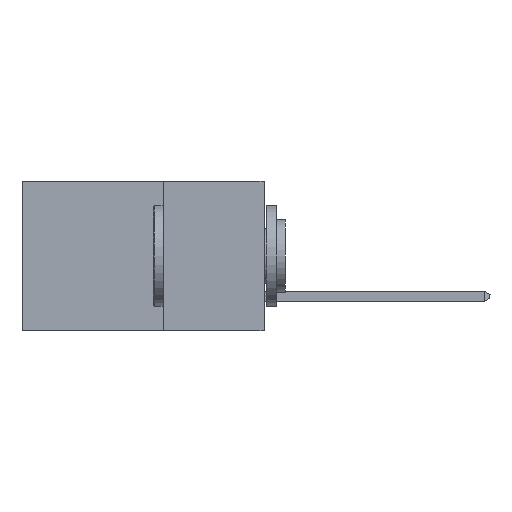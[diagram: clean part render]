
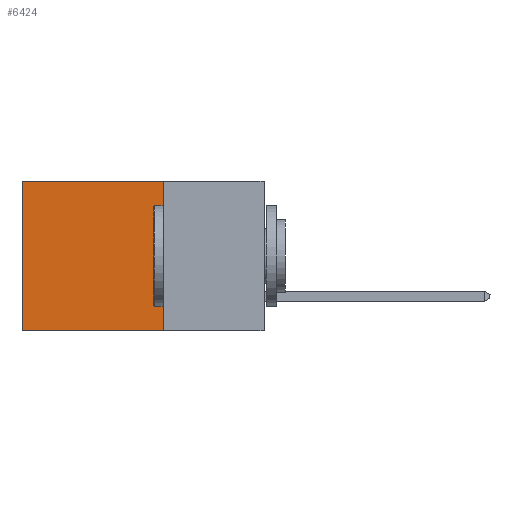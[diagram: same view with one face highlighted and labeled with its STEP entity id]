
A CAD part, left-side view. The second image highlights one B-rep face of the part: STEP entity #6424.
In plain terms, the highlighted planar face has unit normal (-1, 0, 0).
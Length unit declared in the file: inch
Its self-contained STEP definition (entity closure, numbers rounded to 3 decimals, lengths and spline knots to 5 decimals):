
#347 = DIRECTION ( 'NONE',  ( 0., 0., -1. ) ) ;
#1342 = CARTESIAN_POINT ( 'NONE',  ( 0.298, 0.25, -0.37 ) ) ;
#1384 = ORIENTED_EDGE ( 'NONE', *, *, #3387, .F. ) ;
#1698 = CARTESIAN_POINT ( 'NONE',  ( 0.298, 0.25, -0.37 ) ) ;
#1858 = CARTESIAN_POINT ( 'NONE',  ( 0.298, 0.25, 0. ) ) ;
#2007 = VERTEX_POINT ( 'NONE', #1858 ) ;
#2569 = EDGE_CURVE ( 'NONE', #15308, #4708, #13970, .T. ) ;
#2821 = DIRECTION ( 'NONE',  ( 1., 0., 0. ) ) ;
#3040 = EDGE_CURVE ( 'NONE', #11055, #4708, #16139, .T. ) ;
#3202 = DIRECTION ( 'NONE',  ( 0., 0., -1. ) ) ;
#3387 = EDGE_CURVE ( 'NONE', #2007, #11055, #12909, .T. ) ;
#4708 = VERTEX_POINT ( 'NONE', #6383 ) ;
#5152 = CARTESIAN_POINT ( 'NONE',  ( 0.298, 0.6, 0. ) ) ;
#5167 = CARTESIAN_POINT ( 'NONE',  ( 0.298, 0.25, 0. ) ) ;
#5388 = CARTESIAN_POINT ( 'NONE',  ( 0.298, 0.25, 0. ) ) ;
#5919 = VECTOR ( 'NONE', #15610, 39.37008 ) ;
#6383 = CARTESIAN_POINT ( 'NONE',  ( 0.298, 0.6, -0.37 ) ) ;
#6424 = ADVANCED_FACE ( 'NONE', ( #6994 ), #10168, .F. ) ;
#6994 = FACE_OUTER_BOUND ( 'NONE', #8565, .T. ) ;
#7604 = LINE ( 'NONE', #12015, #11972 ) ;
#8565 = EDGE_LOOP ( 'NONE', ( #12563, #10154, #1384, #12296 ) ) ;
#9567 = AXIS2_PLACEMENT_3D ( 'NONE', #5167, #2821, #14130 ) ;
#10154 = ORIENTED_EDGE ( 'NONE', *, *, #3040, .F. ) ;
#10168 = PLANE ( 'NONE',  #9567 ) ;
#10696 = VECTOR ( 'NONE', #3202, 39.37008 ) ;
#11055 = VERTEX_POINT ( 'NONE', #1342 ) ;
#11972 = VECTOR ( 'NONE', #13321, 39.37008 ) ;
#12015 = CARTESIAN_POINT ( 'NONE',  ( 0.298, 0.25, 0. ) ) ;
#12296 = ORIENTED_EDGE ( 'NONE', *, *, #12353, .T. ) ;
#12353 = EDGE_CURVE ( 'NONE', #2007, #15308, #7604, .T. ) ;
#12503 = VECTOR ( 'NONE', #347, 39.37008 ) ;
#12563 = ORIENTED_EDGE ( 'NONE', *, *, #2569, .T. ) ;
#12909 = LINE ( 'NONE', #5388, #12503 ) ;
#13321 = DIRECTION ( 'NONE',  ( 0., 1., 0. ) ) ;
#13388 = CARTESIAN_POINT ( 'NONE',  ( 0.298, 0.6, 0. ) ) ;
#13970 = LINE ( 'NONE', #13388, #10696 ) ;
#14130 = DIRECTION ( 'NONE',  ( 0., 0., -1. ) ) ;
#15308 = VERTEX_POINT ( 'NONE', #5152 ) ;
#15610 = DIRECTION ( 'NONE',  ( 0., 1., 0. ) ) ;
#16139 = LINE ( 'NONE', #1698, #5919 ) ;
